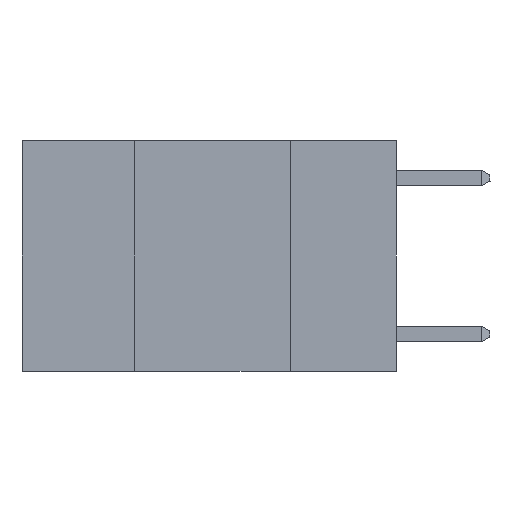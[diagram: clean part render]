
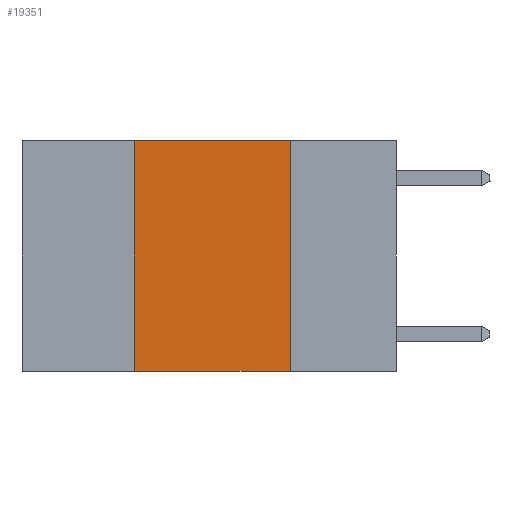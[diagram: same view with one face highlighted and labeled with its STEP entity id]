
A CAD part, left-side view. The second image highlights one B-rep face of the part: STEP entity #19351.
In plain terms, the highlighted planar face has unit normal (-1, 0, 0).
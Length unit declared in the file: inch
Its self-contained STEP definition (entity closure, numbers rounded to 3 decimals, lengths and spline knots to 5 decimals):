
#752 = DIRECTION ( 'NONE',  ( 0., -1., 0. ) ) ;
#2636 = CARTESIAN_POINT ( 'NONE',  ( 0., 0.42, 0. ) ) ;
#2766 = EDGE_LOOP ( 'NONE', ( #10971, #8495, #7791, #4113 ) ) ;
#4059 = CARTESIAN_POINT ( 'NONE',  ( 0., 0.17, 0. ) ) ;
#4113 = ORIENTED_EDGE ( 'NONE', *, *, #21026, .T. ) ;
#4286 = EDGE_CURVE ( 'NONE', #9244, #8930, #15928, .T. ) ;
#5800 = EDGE_CURVE ( 'NONE', #16086, #13918, #7859, .T. ) ;
#5990 = CARTESIAN_POINT ( 'NONE',  ( 0., 0.42, 0. ) ) ;
#7255 = DIRECTION ( 'NONE',  ( 0., -1., 0. ) ) ;
#7791 = ORIENTED_EDGE ( 'NONE', *, *, #4286, .F. ) ;
#7859 = LINE ( 'NONE', #4059, #18848 ) ;
#8296 = LINE ( 'NONE', #26472, #24842 ) ;
#8495 = ORIENTED_EDGE ( 'NONE', *, *, #27809, .F. ) ;
#8702 = DIRECTION ( 'NONE',  ( 1., 0., 0. ) ) ;
#8930 = VERTEX_POINT ( 'NONE', #2636 ) ;
#9244 = VERTEX_POINT ( 'NONE', #27357 ) ;
#10287 = LINE ( 'NONE', #24771, #15435 ) ;
#10553 = DIRECTION ( 'NONE',  ( 0., 0., 1. ) ) ;
#10971 = ORIENTED_EDGE ( 'NONE', *, *, #5800, .F. ) ;
#13128 = CARTESIAN_POINT ( 'NONE',  ( 0., 0.6, 0. ) ) ;
#13918 = VERTEX_POINT ( 'NONE', #25697 ) ;
#15235 = VECTOR ( 'NONE', #10553, 39.37008 ) ;
#15303 = PLANE ( 'NONE',  #22383 ) ;
#15435 = VECTOR ( 'NONE', #752, 39.37008 ) ;
#15928 = LINE ( 'NONE', #5990, #15235 ) ;
#16086 = VERTEX_POINT ( 'NONE', #16168 ) ;
#16168 = CARTESIAN_POINT ( 'NONE',  ( 0., 0.17, 0. ) ) ;
#18848 = VECTOR ( 'NONE', #27843, 39.37008 ) ;
#19246 = FACE_OUTER_BOUND ( 'NONE', #2766, .T. ) ;
#19351 = ADVANCED_FACE ( 'NONE', ( #19246 ), #15303, .F. ) ;
#21026 = EDGE_CURVE ( 'NONE', #9244, #13918, #10287, .T. ) ;
#22383 = AXIS2_PLACEMENT_3D ( 'NONE', #13128, #8702, #23847 ) ;
#23847 = DIRECTION ( 'NONE',  ( 0., 0., -1. ) ) ;
#24771 = CARTESIAN_POINT ( 'NONE',  ( 0., 0.6, -0.37 ) ) ;
#24842 = VECTOR ( 'NONE', #7255, 39.37008 ) ;
#25697 = CARTESIAN_POINT ( 'NONE',  ( 0., 0.17, -0.37 ) ) ;
#26472 = CARTESIAN_POINT ( 'NONE',  ( 0., 0.6, 0. ) ) ;
#27357 = CARTESIAN_POINT ( 'NONE',  ( 0., 0.42, -0.37 ) ) ;
#27809 = EDGE_CURVE ( 'NONE', #8930, #16086, #8296, .T. ) ;
#27843 = DIRECTION ( 'NONE',  ( 0., 0., -1. ) ) ;
